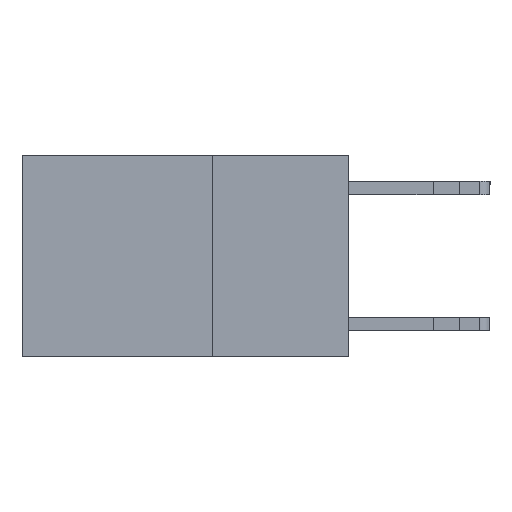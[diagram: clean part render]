
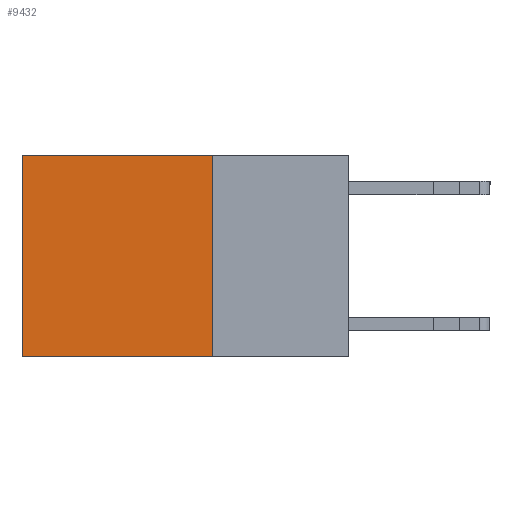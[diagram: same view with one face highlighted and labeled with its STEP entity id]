
A CAD part, left-side view. The second image highlights one B-rep face of the part: STEP entity #9432.
In plain terms, the highlighted planar face has unit normal (-1, 0, 0).
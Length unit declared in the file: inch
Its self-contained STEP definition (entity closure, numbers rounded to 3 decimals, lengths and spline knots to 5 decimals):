
#84 = LINE ( 'NONE', #22338, #15826 ) ;
#618 = EDGE_CURVE ( 'NONE', #2022, #3603, #20500, .T. ) ;
#1028 = ORIENTED_EDGE ( 'NONE', *, *, #7239, .T. ) ;
#1172 = VECTOR ( 'NONE', #7128, 39.37008 ) ;
#2022 = VERTEX_POINT ( 'NONE', #7593 ) ;
#2589 = VECTOR ( 'NONE', #4156, 39.37008 ) ;
#2637 = PLANE ( 'NONE',  #11303 ) ;
#3461 = CARTESIAN_POINT ( 'NONE',  ( 0.2625, 0.6, -0.37 ) ) ;
#3603 = VERTEX_POINT ( 'NONE', #3461 ) ;
#4083 = ORIENTED_EDGE ( 'NONE', *, *, #6497, .F. ) ;
#4156 = DIRECTION ( 'NONE',  ( 0., 1., 0. ) ) ;
#4343 = CARTESIAN_POINT ( 'NONE',  ( 0.2625, 0.6, 0. ) ) ;
#4673 = CARTESIAN_POINT ( 'NONE',  ( 0.2625, 0.25, 0. ) ) ;
#5132 = VERTEX_POINT ( 'NONE', #4343 ) ;
#6497 = EDGE_CURVE ( 'NONE', #16290, #2022, #23018, .T. ) ;
#6634 = CARTESIAN_POINT ( 'NONE',  ( 0.2625, 0.25, 0. ) ) ;
#7128 = DIRECTION ( 'NONE',  ( 0., 1., 0. ) ) ;
#7239 = EDGE_CURVE ( 'NONE', #5132, #3603, #84, .T. ) ;
#7402 = ORIENTED_EDGE ( 'NONE', *, *, #618, .F. ) ;
#7593 = CARTESIAN_POINT ( 'NONE',  ( 0.2625, 0.25, -0.37 ) ) ;
#9432 = ADVANCED_FACE ( 'NONE', ( #19204 ), #2637, .F. ) ;
#9723 = CARTESIAN_POINT ( 'NONE',  ( 0.2625, 0.25, 0. ) ) ;
#10010 = DIRECTION ( 'NONE',  ( 1., 0., 0. ) ) ;
#11303 = AXIS2_PLACEMENT_3D ( 'NONE', #4673, #10010, #17394 ) ;
#11308 = DIRECTION ( 'NONE',  ( 0., 0., -1. ) ) ;
#11992 = CARTESIAN_POINT ( 'NONE',  ( 0.2625, 0.25, 0. ) ) ;
#14619 = ORIENTED_EDGE ( 'NONE', *, *, #20202, .T. ) ;
#15826 = VECTOR ( 'NONE', #11308, 39.37008 ) ;
#15971 = DIRECTION ( 'NONE',  ( 0., 0., -1. ) ) ;
#16059 = LINE ( 'NONE', #6634, #1172 ) ;
#16290 = VERTEX_POINT ( 'NONE', #9723 ) ;
#16853 = CARTESIAN_POINT ( 'NONE',  ( 0.2625, 0.25, -0.37 ) ) ;
#17394 = DIRECTION ( 'NONE',  ( 0., 0., -1. ) ) ;
#18457 = VECTOR ( 'NONE', #15971, 39.37008 ) ;
#19204 = FACE_OUTER_BOUND ( 'NONE', #19255, .T. ) ;
#19255 = EDGE_LOOP ( 'NONE', ( #1028, #7402, #4083, #14619 ) ) ;
#20202 = EDGE_CURVE ( 'NONE', #16290, #5132, #16059, .T. ) ;
#20500 = LINE ( 'NONE', #16853, #2589 ) ;
#22338 = CARTESIAN_POINT ( 'NONE',  ( 0.2625, 0.6, 0. ) ) ;
#23018 = LINE ( 'NONE', #11992, #18457 ) ;
